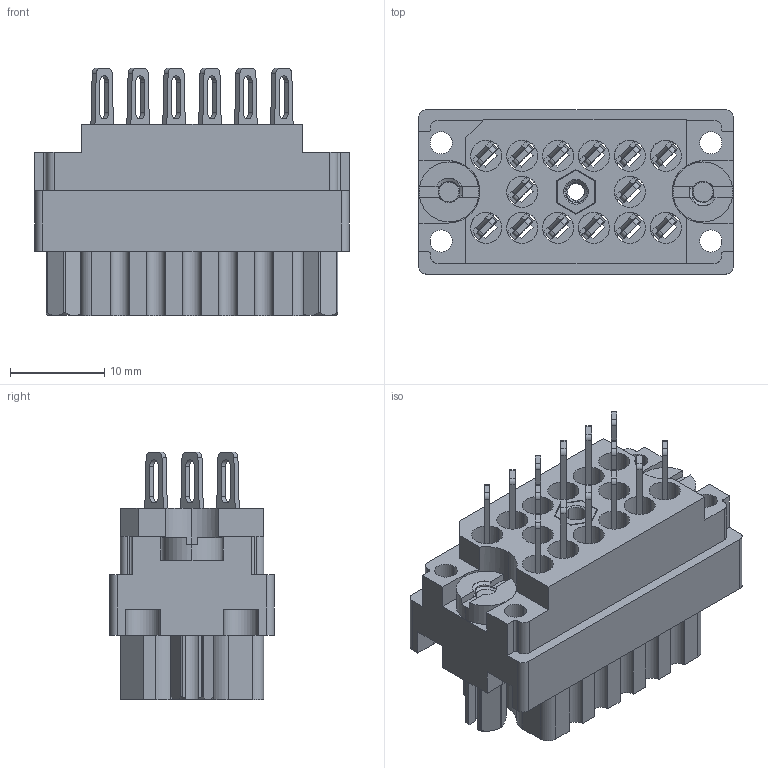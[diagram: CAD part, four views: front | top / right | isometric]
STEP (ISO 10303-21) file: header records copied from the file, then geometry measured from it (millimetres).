
FILE_DESCRIPTION (( 'STEP AP203' ), '1' );
FILE_NAME ('519-014-500-402.STEP', '2020-09-09T17:46:54', ( '' ), ( '' ), 'SwSTEP 2.0', 'SolidWorks 2020', '' );
FILE_SCHEMA (( 'CONFIG_CONTROL_DESIGN' ));
Length unit declared in the file: inch
Products named in the file (7): 516-252-025-100_516-252-025-100; 516-221-020-102_015; 519 Receptacle Insulator_014; 516-252-021-102_014; 519-014-500-402; 516-221-020-102_014; 516-292-001_500 Contact
Assembly tree (20 placements, depth 2):
  519-014-500-402
    519 Receptacle Insulator_014
    516-292-001_500 Contact  x14
    516-252-025-100_516-252-025-100
    516-252-021-102_014  x2
    516-221-020-102_014
    516-221-020-102_015
Bounding box: 33.32 x 17.42 x 26.21 mm (x, y, z)
Volume: 6995.8 mm3; surface area: 10542.6 mm2
Topology: 20 solids, 20 shells, 1770 faces, 5091 edges, 3369 vertices
Faces by surface type: plane 981, cylinder 627, bspline 115, cone 47
Entity records: 32469 total; most frequent: CARTESIAN_POINT 11845, ORIENTED_EDGE 4274, DIRECTION 3914, EDGE_CURVE 2137, VERTEX_POINT 1411, LINE 1338, VECTOR 1338, AXIS2_PLACEMENT_3D 1288
